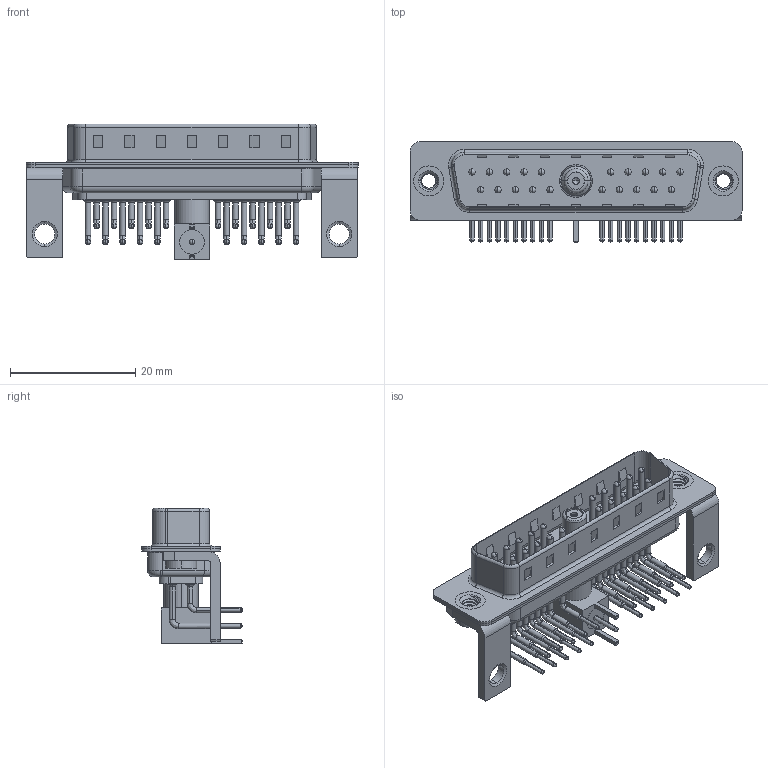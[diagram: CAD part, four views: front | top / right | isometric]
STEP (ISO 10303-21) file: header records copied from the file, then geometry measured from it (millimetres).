
FILE_DESCRIPTION (( 'STEP AP203' ), '1' );
FILE_NAME ('629-21W1640-7NC.STEP', '2022-05-14T02:06:36', ( '' ), ( '' ), 'SwSTEP 2.0', 'SolidWorks 2020', '' );
FILE_SCHEMA (( 'CONFIG_CONTROL_DESIGN' ));
Length unit declared in the file: millimetre
Products named in the file (16): RA Back Shell; 629Combo Stabilizer Bracket; Socket_RA; 629Combo Housing_21W1; Insulator RA Pin; 629Combo Contact Row 1; 629Combo Contact Row 2; 629Combo Shell Front_25 Contacts; 629-21W1640-7NC; Insulator Socket 2; Locking Collar; 629Combo Shell Rear_25 Contacts; 629Combo Threaded Rivet_2; Co-Ax Jack_RA PC Tail; Co-Ax Jack Assy_RA; Insulator Socket
Assembly tree (35 placements, depth 3):
  629-21W1640-7NC
    629Combo Housing_21W1
    629Combo Shell Rear_25 Contacts
    629Combo Shell Front_25 Contacts
    629Combo Threaded Rivet_2  x2
    629Combo Stabilizer Bracket  x2
    Co-Ax Jack Assy_RA
      Co-Ax Jack_RA PC Tail
      Insulator Socket
      Insulator Socket 2
      Locking Collar
      Socket_RA
      RA Back Shell
      Insulator RA Pin
    629Combo Contact Row 1  x10
    629Combo Contact Row 2  x10
Bounding box: 53.05 x 16 x 21.71 mm (x, y, z)
Volume: 3478 mm3; surface area: 9082.2 mm2
Topology: 34 solids, 34 shells, 2776 faces, 7650 edges, 4959 vertices
Faces by surface type: plane 1528, cylinder 948, bspline 127, cone 115, torus 56, sphere 2
Entity records: 30713 total; most frequent: CARTESIAN_POINT 6468, DIRECTION 4824, ORIENTED_EDGE 4422, EDGE_CURVE 2211, AXIS2_PLACEMENT_3D 1772, VERTEX_POINT 1425, VECTOR 1280, LINE 1280
